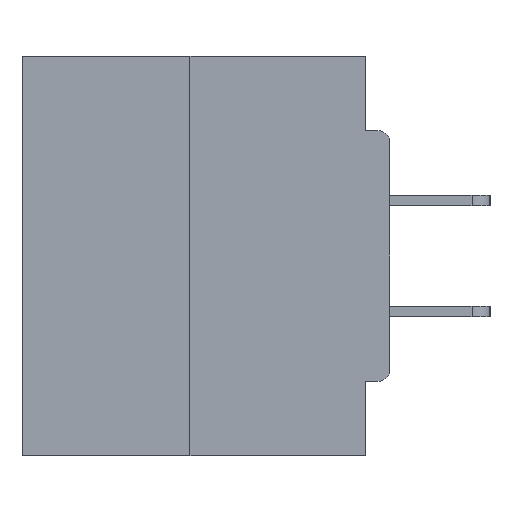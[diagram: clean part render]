
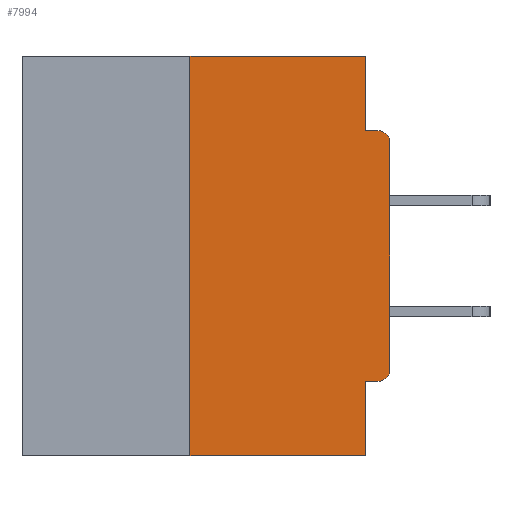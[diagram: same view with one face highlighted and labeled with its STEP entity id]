
A CAD part, left-side view. The second image highlights one B-rep face of the part: STEP entity #7994.
In plain terms, the highlighted planar face has unit normal (-1, 0, 0).
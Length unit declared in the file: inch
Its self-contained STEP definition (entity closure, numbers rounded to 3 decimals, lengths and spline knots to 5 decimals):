
#498 = VECTOR ( 'NONE', #26364, 39.37008 ) ;
#502 = DIRECTION ( 'NONE',  ( 0., 1., 0. ) ) ;
#981 = VECTOR ( 'NONE', #27047, 39.37008 ) ;
#1182 = AXIS2_PLACEMENT_3D ( 'NONE', #16983, #22756, #8513 ) ;
#1407 = LINE ( 'NONE', #4058, #981 ) ;
#1676 = AXIS2_PLACEMENT_3D ( 'NONE', #10994, #36182, #5005 ) ;
#1980 = CARTESIAN_POINT ( 'NONE',  ( 0., 0., -0.1085 ) ) ;
#2060 = CARTESIAN_POINT ( 'NONE',  ( 0., 0.25, 0. ) ) ;
#2150 = CARTESIAN_POINT ( 'NONE',  ( 0., 0.031, 0. ) ) ;
#2312 = CARTESIAN_POINT ( 'NONE',  ( 0., 0.015, -0.0935 ) ) ;
#2461 = ORIENTED_EDGE ( 'NONE', *, *, #13478, .F. ) ;
#2851 = LINE ( 'NONE', #2150, #7329 ) ;
#3177 = LINE ( 'NONE', #23982, #498 ) ;
#4058 = CARTESIAN_POINT ( 'NONE',  ( 0., 0.46, 0. ) ) ;
#5005 = DIRECTION ( 'NONE',  ( 0., 0., -1. ) ) ;
#5123 = CARTESIAN_POINT ( 'NONE',  ( 0., 0.25, -0.5 ) ) ;
#6019 = VECTOR ( 'NONE', #7661, 39.37008 ) ;
#6393 = VECTOR ( 'NONE', #35306, 39.37008 ) ;
#6711 = EDGE_CURVE ( 'NONE', #10806, #31542, #9825, .T. ) ;
#6893 = LINE ( 'NONE', #31350, #33595 ) ;
#7084 = CARTESIAN_POINT ( 'NONE',  ( 0., 0.015, -0.4065 ) ) ;
#7329 = VECTOR ( 'NONE', #30824, 39.37008 ) ;
#7661 = DIRECTION ( 'NONE',  ( 0., 0., 1. ) ) ;
#7994 = ADVANCED_FACE ( 'NONE', ( #29348 ), #22135, .F. ) ;
#8513 = DIRECTION ( 'NONE',  ( 0., 0., -1. ) ) ;
#8576 = EDGE_CURVE ( 'NONE', #26585, #34305, #28924, .T. ) ;
#9008 = ORIENTED_EDGE ( 'NONE', *, *, #13813, .F. ) ;
#9353 = ORIENTED_EDGE ( 'NONE', *, *, #6711, .T. ) ;
#9825 = CIRCLE ( 'NONE', #1182, 0.015 ) ;
#10235 = CARTESIAN_POINT ( 'NONE',  ( 0., 0.031, -0.5 ) ) ;
#10505 = EDGE_CURVE ( 'NONE', #26047, #22095, #11353, .T. ) ;
#10806 = VERTEX_POINT ( 'NONE', #1980 ) ;
#10887 = LINE ( 'NONE', #21269, #6393 ) ;
#10994 = CARTESIAN_POINT ( 'NONE',  ( 0., 0.46, 0. ) ) ;
#11353 = LINE ( 'NONE', #29441, #22546 ) ;
#13149 = ORIENTED_EDGE ( 'NONE', *, *, #15289, .T. ) ;
#13478 = EDGE_CURVE ( 'NONE', #24016, #29165, #2851, .T. ) ;
#13638 = DIRECTION ( 'NONE',  ( 0., 0., 1. ) ) ;
#13813 = EDGE_CURVE ( 'NONE', #22095, #35815, #10887, .T. ) ;
#15289 = EDGE_CURVE ( 'NONE', #26585, #35815, #3177, .T. ) ;
#16983 = CARTESIAN_POINT ( 'NONE',  ( 0., 0.015, -0.1085 ) ) ;
#16987 = EDGE_CURVE ( 'NONE', #26047, #34933, #20979, .T. ) ;
#17000 = DIRECTION ( 'NONE',  ( -1., 0., 0. ) ) ;
#17226 = ORIENTED_EDGE ( 'NONE', *, *, #10505, .F. ) ;
#17303 = ORIENTED_EDGE ( 'NONE', *, *, #8576, .F. ) ;
#17307 = EDGE_LOOP ( 'NONE', ( #36615, #17303, #13149, #9008, #17226, #18405, #33188, #9353, #29387, #2461 ) ) ;
#17492 = CARTESIAN_POINT ( 'NONE',  ( 0., 0.031, 0. ) ) ;
#18405 = ORIENTED_EDGE ( 'NONE', *, *, #16987, .T. ) ;
#19145 = EDGE_CURVE ( 'NONE', #34305, #24016, #1407, .T. ) ;
#19660 = CARTESIAN_POINT ( 'NONE',  ( 0., 0.015, -0.3915 ) ) ;
#20979 = CIRCLE ( 'NONE', #28185, 0.015 ) ;
#21269 = CARTESIAN_POINT ( 'NONE',  ( 0., 0.031, -0.5 ) ) ;
#22095 = VERTEX_POINT ( 'NONE', #31938 ) ;
#22135 = PLANE ( 'NONE',  #1676 ) ;
#22546 = VECTOR ( 'NONE', #502, 39.37008 ) ;
#22756 = DIRECTION ( 'NONE',  ( -1., 0., 0. ) ) ;
#23353 = EDGE_CURVE ( 'NONE', #29165, #31542, #6893, .T. ) ;
#23982 = CARTESIAN_POINT ( 'NONE',  ( 0., 0.46, -0.5 ) ) ;
#24016 = VERTEX_POINT ( 'NONE', #17492 ) ;
#24901 = CARTESIAN_POINT ( 'NONE',  ( 0., 0., 0. ) ) ;
#26047 = VERTEX_POINT ( 'NONE', #7084 ) ;
#26364 = DIRECTION ( 'NONE',  ( 0., -1., 0. ) ) ;
#26585 = VERTEX_POINT ( 'NONE', #5123 ) ;
#27047 = DIRECTION ( 'NONE',  ( 0., -1., 0. ) ) ;
#27455 = CARTESIAN_POINT ( 'NONE',  ( 0., 0., -0.3915 ) ) ;
#28151 = DIRECTION ( 'NONE',  ( 0., 0., -1. ) ) ;
#28185 = AXIS2_PLACEMENT_3D ( 'NONE', #19660, #17000, #28151 ) ;
#28755 = DIRECTION ( 'NONE',  ( 0., -1., 0. ) ) ;
#28924 = LINE ( 'NONE', #2060, #32018 ) ;
#29165 = VERTEX_POINT ( 'NONE', #30205 ) ;
#29348 = FACE_OUTER_BOUND ( 'NONE', #17307, .T. ) ;
#29387 = ORIENTED_EDGE ( 'NONE', *, *, #23353, .F. ) ;
#29441 = CARTESIAN_POINT ( 'NONE',  ( 0., 0., -0.4065 ) ) ;
#30205 = CARTESIAN_POINT ( 'NONE',  ( 0., 0.031, -0.0935 ) ) ;
#30824 = DIRECTION ( 'NONE',  ( 0., 0., -1. ) ) ;
#31350 = CARTESIAN_POINT ( 'NONE',  ( 0., 0., -0.0935 ) ) ;
#31542 = VERTEX_POINT ( 'NONE', #2312 ) ;
#31938 = CARTESIAN_POINT ( 'NONE',  ( 0., 0.031, -0.4065 ) ) ;
#32018 = VECTOR ( 'NONE', #13638, 39.37008 ) ;
#33063 = CARTESIAN_POINT ( 'NONE',  ( 0., 0.25, 0. ) ) ;
#33188 = ORIENTED_EDGE ( 'NONE', *, *, #36475, .T. ) ;
#33595 = VECTOR ( 'NONE', #28755, 39.37008 ) ;
#34305 = VERTEX_POINT ( 'NONE', #33063 ) ;
#34933 = VERTEX_POINT ( 'NONE', #27455 ) ;
#35306 = DIRECTION ( 'NONE',  ( 0., 0., -1. ) ) ;
#35815 = VERTEX_POINT ( 'NONE', #10235 ) ;
#36182 = DIRECTION ( 'NONE',  ( 1., 0., 0. ) ) ;
#36374 = LINE ( 'NONE', #24901, #6019 ) ;
#36475 = EDGE_CURVE ( 'NONE', #34933, #10806, #36374, .T. ) ;
#36615 = ORIENTED_EDGE ( 'NONE', *, *, #19145, .F. ) ;
